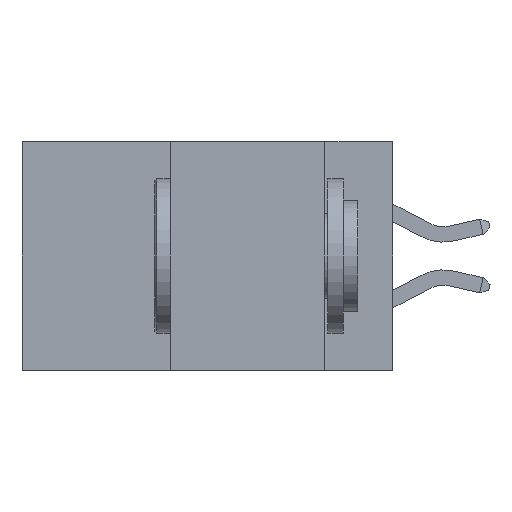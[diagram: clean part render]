
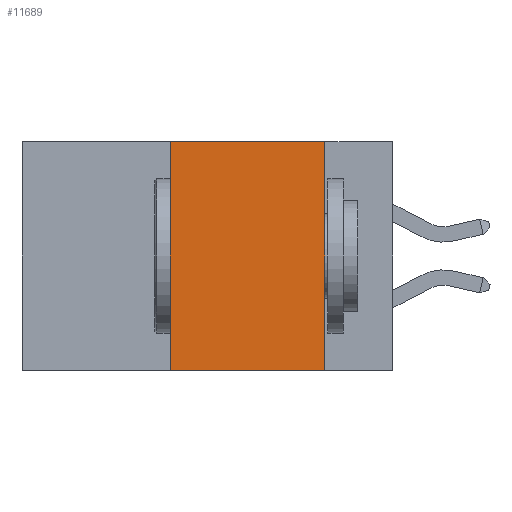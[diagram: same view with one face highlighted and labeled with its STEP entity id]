
A CAD part, left-side view. The second image highlights one B-rep face of the part: STEP entity #11689.
In plain terms, the highlighted planar face has unit normal (-1, 0, 0).
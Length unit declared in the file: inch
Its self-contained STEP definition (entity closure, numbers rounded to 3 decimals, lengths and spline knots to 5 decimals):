
#172 = CARTESIAN_POINT ( 'NONE',  ( 0., 0.6, -0.37 ) ) ;
#1072 = VERTEX_POINT ( 'NONE', #6270 ) ;
#1247 = DIRECTION ( 'NONE',  ( 1., 0., 0. ) ) ;
#1370 = AXIS2_PLACEMENT_3D ( 'NONE', #2609, #1247, #11405 ) ;
#1449 = CARTESIAN_POINT ( 'NONE',  ( 0., 0.36, -0.37 ) ) ;
#1460 = LINE ( 'NONE', #2412, #3818 ) ;
#2412 = CARTESIAN_POINT ( 'NONE',  ( 0., 0.6, 0. ) ) ;
#2609 = CARTESIAN_POINT ( 'NONE',  ( 0., 0.6, 0. ) ) ;
#3082 = VERTEX_POINT ( 'NONE', #4279 ) ;
#3098 = VERTEX_POINT ( 'NONE', #1449 ) ;
#3818 = VECTOR ( 'NONE', #9471, 39.37008 ) ;
#4279 = CARTESIAN_POINT ( 'NONE',  ( 0., 0.11, -0.37 ) ) ;
#4541 = VECTOR ( 'NONE', #10199, 39.37008 ) ;
#4771 = DIRECTION ( 'NONE',  ( 0., 0., 1. ) ) ;
#5061 = EDGE_CURVE ( 'NONE', #1072, #3082, #9584, .T. ) ;
#5073 = EDGE_CURVE ( 'NONE', #3098, #7303, #10043, .T. ) ;
#5179 = ORIENTED_EDGE ( 'NONE', *, *, #9418, .T. ) ;
#6270 = CARTESIAN_POINT ( 'NONE',  ( 0., 0.11, 0. ) ) ;
#6797 = ORIENTED_EDGE ( 'NONE', *, *, #11982, .F. ) ;
#7208 = LINE ( 'NONE', #172, #4541 ) ;
#7303 = VERTEX_POINT ( 'NONE', #9248 ) ;
#7316 = DIRECTION ( 'NONE',  ( 0., 0., -1. ) ) ;
#7730 = EDGE_LOOP ( 'NONE', ( #9513, #6797, #9087, #5179 ) ) ;
#9087 = ORIENTED_EDGE ( 'NONE', *, *, #5073, .F. ) ;
#9248 = CARTESIAN_POINT ( 'NONE',  ( 0., 0.36, 0. ) ) ;
#9252 = VECTOR ( 'NONE', #7316, 39.37008 ) ;
#9268 = FACE_OUTER_BOUND ( 'NONE', #7730, .T. ) ;
#9418 = EDGE_CURVE ( 'NONE', #3098, #3082, #7208, .T. ) ;
#9471 = DIRECTION ( 'NONE',  ( 0., -1., 0. ) ) ;
#9513 = ORIENTED_EDGE ( 'NONE', *, *, #5061, .F. ) ;
#9584 = LINE ( 'NONE', #12508, #9252 ) ;
#10043 = LINE ( 'NONE', #11062, #11643 ) ;
#10199 = DIRECTION ( 'NONE',  ( 0., -1., 0. ) ) ;
#11062 = CARTESIAN_POINT ( 'NONE',  ( 0., 0.36, 0. ) ) ;
#11405 = DIRECTION ( 'NONE',  ( 0., 0., -1. ) ) ;
#11643 = VECTOR ( 'NONE', #4771, 39.37008 ) ;
#11689 = ADVANCED_FACE ( 'NONE', ( #9268 ), #11804, .F. ) ;
#11804 = PLANE ( 'NONE',  #1370 ) ;
#11982 = EDGE_CURVE ( 'NONE', #7303, #1072, #1460, .T. ) ;
#12508 = CARTESIAN_POINT ( 'NONE',  ( 0., 0.11, 0. ) ) ;
